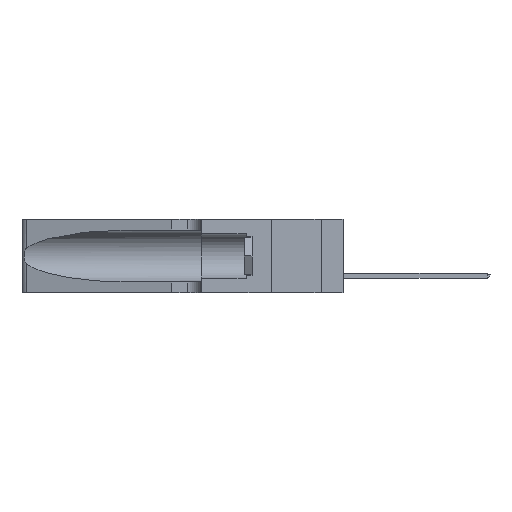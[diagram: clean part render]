
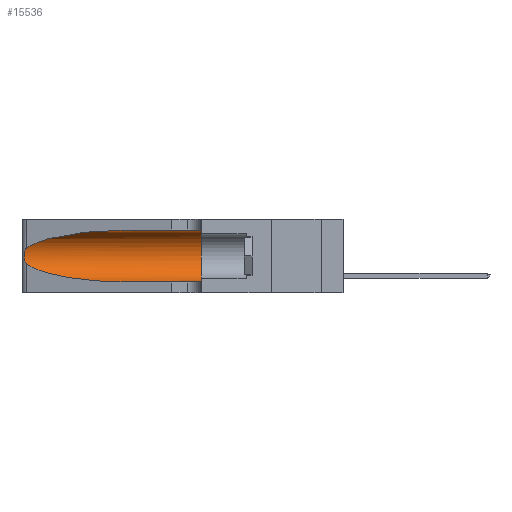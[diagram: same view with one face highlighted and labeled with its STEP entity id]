
A CAD part, left-side view. The second image highlights one B-rep face of the part: STEP entity #15536.
In plain terms, the highlighted cylindrical face has radius 3.308 mm (diameter 6.617 mm), a partial arc.
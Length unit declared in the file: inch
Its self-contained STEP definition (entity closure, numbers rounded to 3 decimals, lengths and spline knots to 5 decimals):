
#292 = CARTESIAN_POINT ( 'NONE',  ( 0.18966, 0.96281, 0.05475 ) ) ;
#482 = DIRECTION ( 'NONE',  ( 0., 0., -1. ) ) ;
#582 = CARTESIAN_POINT ( 'NONE',  ( 0.25555, 1.22993, 0.14849 ) ) ;
#819 = AXIS2_PLACEMENT_3D ( 'NONE', #4291, #1877, #27460 ) ;
#842 = CARTESIAN_POINT ( 'NONE',  ( 0.1305, 0.72297, 0.31525 ) ) ;
#1877 = DIRECTION ( 'NONE',  ( 0., 1., 0. ) ) ;
#2657 = CARTESIAN_POINT ( 'NONE',  ( 0.18966, 0.96281, 0.31525 ) ) ;
#2711 = ORIENTED_EDGE ( 'NONE', *, *, #3685, .F. ) ;
#3236 = ORIENTED_EDGE ( 'NONE', *, *, #24509, .T. ) ;
#3605 = LINE ( 'NONE', #22719, #7599 ) ;
#3641 = CARTESIAN_POINT ( 'NONE',  ( 0.1305, 1.61858, 0.185 ) ) ;
#3685 = EDGE_CURVE ( 'NONE', #32769, #28134, #3605, .T. ) ;
#3850 = CARTESIAN_POINT ( 'NONE',  ( 0.25487, 1.22718, 0.14631 ) ) ;
#4291 = CARTESIAN_POINT ( 'NONE',  ( 0.1305, 0.35, 0.185 ) ) ;
#5236 = CARTESIAN_POINT ( 'NONE',  ( 0.1305, 0.35, 0.05475 ) ) ;
#5871 = CARTESIAN_POINT ( 'NONE',  ( 0.2373, 1.15595, 0.28018 ) ) ;
#6207 =( BOUNDED_CURVE ( )  B_SPLINE_CURVE ( 3, ( #40833, #2657, #5871, #34742 ),
 .UNSPECIFIED., .F., .T. ) 
 B_SPLINE_CURVE_WITH_KNOTS ( ( 4, 4 ),
 ( 1.5708, 2.84003 ),
 .UNSPECIFIED. ) 
 CURVE ( )  GEOMETRIC_REPRESENTATION_ITEM ( )  RATIONAL_B_SPLINE_CURVE ( ( 1., 0.87, 0.87, 1. ) ) 
 REPRESENTATION_ITEM ( '' )  );
#6251 = DIRECTION ( 'NONE',  ( 0., -1., 0. ) ) ;
#6597 = CYLINDRICAL_SURFACE ( 'NONE', #10949, 0.13025 ) ;
#7599 = VECTOR ( 'NONE', #6251, 39.37008 ) ;
#8634 = CARTESIAN_POINT ( 'NONE',  ( 0.25487, 1.22718, 0.22369 ) ) ;
#8731 = B_SPLINE_CURVE_WITH_KNOTS ( 'NONE', 3,
 ( #8634, #37494, #31535, #34989, #41101, #31663, #22337, #25544, #35244, #29008, #32326, #29274, #582, #3850 ),
 .UNSPECIFIED., .F., .F.,
 ( 4, 2, 2, 2, 2, 2, 4 ),
 ( 0., 0.00027, 0.00053, 0.00107, 0.0016, 0.00187, 0.00214 ),
 .UNSPECIFIED. ) ;
#9586 = EDGE_CURVE ( 'NONE', #32769, #21066, #6207, .T. ) ;
#9975 = CARTESIAN_POINT ( 'NONE',  ( 0.25487, 1.22718, 0.14631 ) ) ;
#10677 = CARTESIAN_POINT ( 'NONE',  ( 0.1305, 0.35, 0.31525 ) ) ;
#10949 = AXIS2_PLACEMENT_3D ( 'NONE', #3641, #13256, #482 ) ;
#12046 = LINE ( 'NONE', #14588, #28580 ) ;
#13188 = CARTESIAN_POINT ( 'NONE',  ( 0.2373, 1.15595, 0.08982 ) ) ;
#13256 = DIRECTION ( 'NONE',  ( 0., -1., 0. ) ) ;
#14588 = CARTESIAN_POINT ( 'NONE',  ( 0.1305, 1.61858, 0.05475 ) ) ;
#15256 = EDGE_CURVE ( 'NONE', #21066, #31405, #8731, .T. ) ;
#15536 = ADVANCED_FACE ( 'NONE', ( #37831 ), #6597, .F. ) ;
#16580 = EDGE_LOOP ( 'NONE', ( #28245, #21206, #26579, #3236, #37437, #2711 ) ) ;
#20960 = CARTESIAN_POINT ( 'NONE',  ( 0.1305, 0.72297, 0.05475 ) ) ;
#21066 = VERTEX_POINT ( 'NONE', #37516 ) ;
#21206 = ORIENTED_EDGE ( 'NONE', *, *, #15256, .T. ) ;
#22337 = CARTESIAN_POINT ( 'NONE',  ( 0.26075, 1.23896, 0.19203 ) ) ;
#22433 = CIRCLE ( 'NONE', #819, 0.13025 ) ;
#22719 = CARTESIAN_POINT ( 'NONE',  ( 0.1305, 1.61858, 0.31525 ) ) ;
#23423 = VERTEX_POINT ( 'NONE', #20960 ) ;
#24499 = VERTEX_POINT ( 'NONE', #5236 ) ;
#24509 = EDGE_CURVE ( 'NONE', #23423, #24499, #12046, .T. ) ;
#25544 = CARTESIAN_POINT ( 'NONE',  ( 0.26075, 1.23896, 0.178 ) ) ;
#26579 = ORIENTED_EDGE ( 'NONE', *, *, #37813, .T. ) ;
#26642 =( BOUNDED_CURVE ( )  B_SPLINE_CURVE ( 3, ( #9975, #13188, #292, #29379 ),
 .UNSPECIFIED., .F., .F. ) 
 B_SPLINE_CURVE_WITH_KNOTS ( ( 4, 4 ),
 ( 3.44316, 4.71239 ),
 .UNSPECIFIED. ) 
 CURVE ( )  GEOMETRIC_REPRESENTATION_ITEM ( )  RATIONAL_B_SPLINE_CURVE ( ( 1., 0.87, 0.87, 1. ) ) 
 REPRESENTATION_ITEM ( '' )  );
#27460 = DIRECTION ( 'NONE',  ( 0., 0., 1. ) ) ;
#28030 = CARTESIAN_POINT ( 'NONE',  ( 0.25487, 1.22718, 0.14631 ) ) ;
#28134 = VERTEX_POINT ( 'NONE', #10677 ) ;
#28245 = ORIENTED_EDGE ( 'NONE', *, *, #9586, .T. ) ;
#28580 = VECTOR ( 'NONE', #40063, 39.37008 ) ;
#29008 = CARTESIAN_POINT ( 'NONE',  ( 0.25856, 1.23593, 0.16098 ) ) ;
#29274 = CARTESIAN_POINT ( 'NONE',  ( 0.25639, 1.23186, 0.15144 ) ) ;
#29379 = CARTESIAN_POINT ( 'NONE',  ( 0.1305, 0.72297, 0.05475 ) ) ;
#31405 = VERTEX_POINT ( 'NONE', #28030 ) ;
#31535 = CARTESIAN_POINT ( 'NONE',  ( 0.25639, 1.23184, 0.21858 ) ) ;
#31663 = CARTESIAN_POINT ( 'NONE',  ( 0.26018, 1.23835, 0.19895 ) ) ;
#32326 = CARTESIAN_POINT ( 'NONE',  ( 0.25789, 1.23486, 0.15765 ) ) ;
#32769 = VERTEX_POINT ( 'NONE', #842 ) ;
#34742 = CARTESIAN_POINT ( 'NONE',  ( 0.25487, 1.22718, 0.22369 ) ) ;
#34989 = CARTESIAN_POINT ( 'NONE',  ( 0.25787, 1.23484, 0.2124 ) ) ;
#35244 = CARTESIAN_POINT ( 'NONE',  ( 0.26017, 1.23833, 0.17102 ) ) ;
#36506 = EDGE_CURVE ( 'NONE', #28134, #24499, #22433, .T. ) ;
#37437 = ORIENTED_EDGE ( 'NONE', *, *, #36506, .F. ) ;
#37494 = CARTESIAN_POINT ( 'NONE',  ( 0.25555, 1.22994, 0.2215 ) ) ;
#37516 = CARTESIAN_POINT ( 'NONE',  ( 0.25487, 1.22718, 0.22369 ) ) ;
#37813 = EDGE_CURVE ( 'NONE', #31405, #23423, #26642, .T. ) ;
#37831 = FACE_OUTER_BOUND ( 'NONE', #16580, .T. ) ;
#40063 = DIRECTION ( 'NONE',  ( 0., -1., 0. ) ) ;
#40833 = CARTESIAN_POINT ( 'NONE',  ( 0.1305, 0.72297, 0.31525 ) ) ;
#41101 = CARTESIAN_POINT ( 'NONE',  ( 0.25854, 1.2359, 0.20912 ) ) ;
